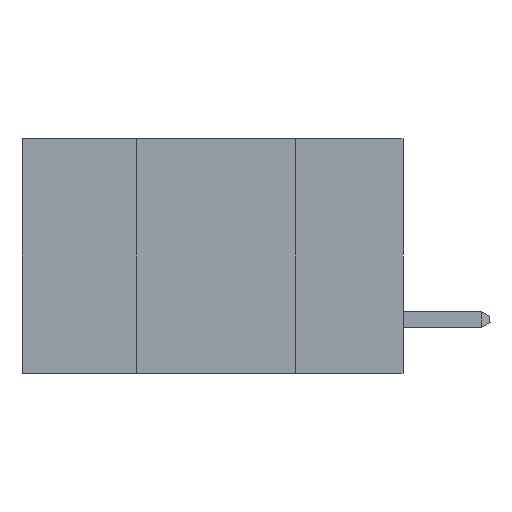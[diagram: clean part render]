
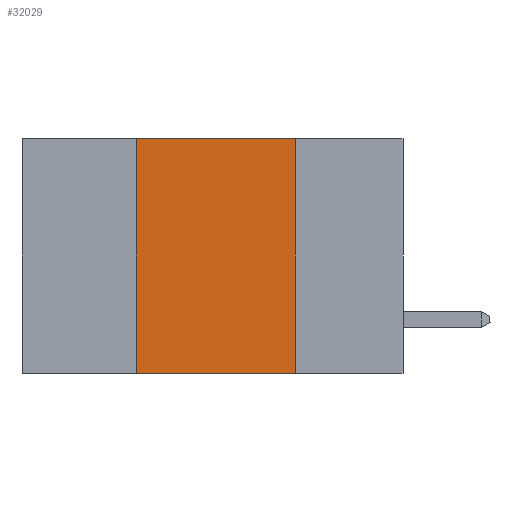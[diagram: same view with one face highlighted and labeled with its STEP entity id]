
A CAD part, left-side view. The second image highlights one B-rep face of the part: STEP entity #32029.
In plain terms, the highlighted planar face has unit normal (-1, 0, 0).
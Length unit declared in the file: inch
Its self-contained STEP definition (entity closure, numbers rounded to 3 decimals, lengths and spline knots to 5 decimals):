
#5 = LINE ( 'NONE', #24862, #24243 ) ;
#664 = CARTESIAN_POINT ( 'NONE',  ( 0., 0.6, 0. ) ) ;
#2481 = EDGE_LOOP ( 'NONE', ( #9294, #20945, #17213, #12059 ) ) ;
#3175 = LINE ( 'NONE', #664, #5441 ) ;
#3355 = VECTOR ( 'NONE', #29849, 39.37008 ) ;
#4005 = DIRECTION ( 'NONE',  ( 0., -1., 0. ) ) ;
#5441 = VECTOR ( 'NONE', #11946, 39.37008 ) ;
#6280 = CARTESIAN_POINT ( 'NONE',  ( 0., 0.6, -0.37 ) ) ;
#6720 = CARTESIAN_POINT ( 'NONE',  ( 0., 0.17, 0. ) ) ;
#6776 = FACE_OUTER_BOUND ( 'NONE', #2481, .T. ) ;
#6994 = EDGE_CURVE ( 'NONE', #10199, #33977, #3175, .T. ) ;
#7729 = VERTEX_POINT ( 'NONE', #26930 ) ;
#9294 = ORIENTED_EDGE ( 'NONE', *, *, #16767, .F. ) ;
#10199 = VERTEX_POINT ( 'NONE', #10297 ) ;
#10297 = CARTESIAN_POINT ( 'NONE',  ( 0., 0.42, 0. ) ) ;
#11946 = DIRECTION ( 'NONE',  ( 0., -1., 0. ) ) ;
#12059 = ORIENTED_EDGE ( 'NONE', *, *, #18549, .T. ) ;
#13746 = CARTESIAN_POINT ( 'NONE',  ( 0., 0.42, -0.37 ) ) ;
#14547 = VECTOR ( 'NONE', #4005, 39.37008 ) ;
#16308 = DIRECTION ( 'NONE',  ( 0., 0., -1. ) ) ;
#16767 = EDGE_CURVE ( 'NONE', #33977, #7729, #5, .T. ) ;
#17144 = CARTESIAN_POINT ( 'NONE',  ( 0., 0.6, 0. ) ) ;
#17213 = ORIENTED_EDGE ( 'NONE', *, *, #27206, .F. ) ;
#18549 = EDGE_CURVE ( 'NONE', #32929, #7729, #31209, .T. ) ;
#20945 = ORIENTED_EDGE ( 'NONE', *, *, #6994, .F. ) ;
#23269 = DIRECTION ( 'NONE',  ( 1., 0., 0. ) ) ;
#24243 = VECTOR ( 'NONE', #16308, 39.37008 ) ;
#24862 = CARTESIAN_POINT ( 'NONE',  ( 0., 0.17, 0. ) ) ;
#26175 = DIRECTION ( 'NONE',  ( 0., 0., -1. ) ) ;
#26930 = CARTESIAN_POINT ( 'NONE',  ( 0., 0.17, -0.37 ) ) ;
#27206 = EDGE_CURVE ( 'NONE', #32929, #10199, #30824, .T. ) ;
#29849 = DIRECTION ( 'NONE',  ( 0., 0., 1. ) ) ;
#30824 = LINE ( 'NONE', #33037, #3355 ) ;
#31209 = LINE ( 'NONE', #6280, #14547 ) ;
#31265 = PLANE ( 'NONE',  #32102 ) ;
#32029 = ADVANCED_FACE ( 'NONE', ( #6776 ), #31265, .F. ) ;
#32102 = AXIS2_PLACEMENT_3D ( 'NONE', #17144, #23269, #26175 ) ;
#32929 = VERTEX_POINT ( 'NONE', #13746 ) ;
#33037 = CARTESIAN_POINT ( 'NONE',  ( 0., 0.42, 0. ) ) ;
#33977 = VERTEX_POINT ( 'NONE', #6720 ) ;
